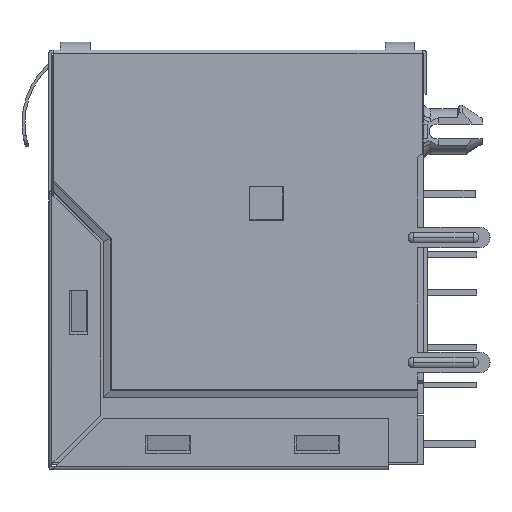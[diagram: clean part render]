
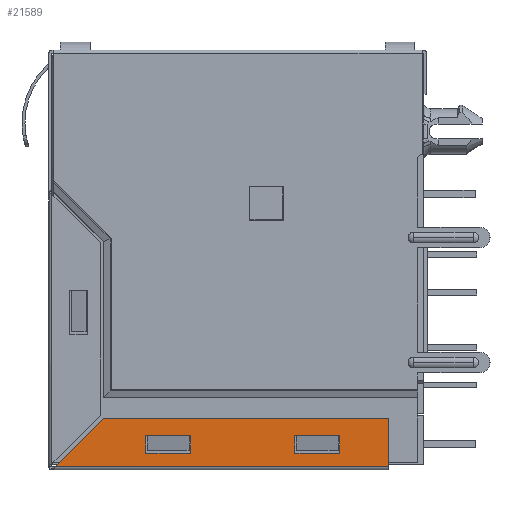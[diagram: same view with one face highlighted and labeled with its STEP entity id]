
A CAD part, left-side view. The second image highlights one B-rep face of the part: STEP entity #21589.
In plain terms, the highlighted planar face has unit normal (-1, 0, 0).
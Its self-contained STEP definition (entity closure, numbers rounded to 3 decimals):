
#802 = FACE_BOUND ( 'NONE', #19686, .T. ) ;
#1521 = VERTEX_POINT ( 'NONE', #7287 ) ;
#1597 = CARTESIAN_POINT ( 'NONE',  ( -31.88, 3.165, -25.58 ) ) ;
#2437 = ORIENTED_EDGE ( 'NONE', *, *, #51071, .T. ) ;
#3403 = CARTESIAN_POINT ( 'NONE',  ( -31.88, -6.835, -25.58 ) ) ;
#3561 = CARTESIAN_POINT ( 'NONE',  ( -31.88, -10.135, -27.67 ) ) ;
#5840 = CARTESIAN_POINT ( 'NONE',  ( -31.88, -10.135, -24.43 ) ) ;
#6438 = B_SPLINE_CURVE_WITH_KNOTS ( 'NONE', 1,
 ( #54370, #48683 ),
 .UNSPECIFIED., .F., .F.,
 ( 2, 2 ),
 ( 0., 1. ),
 .UNSPECIFIED. ) ;
#7287 = CARTESIAN_POINT ( 'NONE',  ( -31.88, -6.835, -26.78 ) ) ;
#7447 = B_SPLINE_CURVE_WITH_KNOTS ( 'NONE', 1,
 ( #21721, #28729 ),
 .UNSPECIFIED., .F., .F.,
 ( 2, 2 ),
 ( 0., 1. ),
 .UNSPECIFIED. ) ;
#9103 = CARTESIAN_POINT ( 'NONE',  ( -31.88, -6.835, -26.78 ) ) ;
#10113 = ORIENTED_EDGE ( 'NONE', *, *, #70867, .T. ) ;
#10382 = VERTEX_POINT ( 'NONE', #18526 ) ;
#10757 = VERTEX_POINT ( 'NONE', #53356 ) ;
#12150 = EDGE_LOOP ( 'NONE', ( #12982, #2437, #44208, #40241 ) ) ;
#12982 = ORIENTED_EDGE ( 'NONE', *, *, #63457, .T. ) ;
#13313 = CARTESIAN_POINT ( 'NONE',  ( -31.88, 6.165, -25.58 ) ) ;
#13814 = VERTEX_POINT ( 'NONE', #75172 ) ;
#15710 = CARTESIAN_POINT ( 'NONE',  ( -31.88, 9.005, -24.43 ) ) ;
#16967 = B_SPLINE_CURVE_WITH_KNOTS ( 'NONE', 1,
 ( #24337, #18397 ),
 .UNSPECIFIED., .F., .F.,
 ( 2, 2 ),
 ( 0., 1. ),
 .UNSPECIFIED. ) ;
#18397 = CARTESIAN_POINT ( 'NONE',  ( -31.88, -3.835, -26.78 ) ) ;
#18526 = CARTESIAN_POINT ( 'NONE',  ( -31.88, 12.245, -27.67 ) ) ;
#19686 = EDGE_LOOP ( 'NONE', ( #55014, #79416, #56093, #74237 ) ) ;
#20128 = CARTESIAN_POINT ( 'NONE',  ( -31.88, 6.165, -25.58 ) ) ;
#20222 = DIRECTION ( 'NONE',  ( -1., 0., 0. ) ) ;
#21165 = VERTEX_POINT ( 'NONE', #30728 ) ;
#21589 = ADVANCED_FACE ( 'NONE', ( #76416, #802, #34754 ), #44592, .T. ) ;
#21721 = CARTESIAN_POINT ( 'NONE',  ( -31.88, -3.835, -26.78 ) ) ;
#24337 = CARTESIAN_POINT ( 'NONE',  ( -31.88, -6.835, -26.78 ) ) ;
#25726 = VERTEX_POINT ( 'NONE', #26271 ) ;
#25918 = ORIENTED_EDGE ( 'NONE', *, *, #73327, .T. ) ;
#26271 = CARTESIAN_POINT ( 'NONE',  ( -31.88, -3.835, -26.78 ) ) ;
#28687 = EDGE_CURVE ( 'NONE', #77531, #10382, #40807, .T. ) ;
#28729 = CARTESIAN_POINT ( 'NONE',  ( -31.88, -3.835, -25.58 ) ) ;
#29521 = EDGE_LOOP ( 'NONE', ( #41422, #25918, #47184, #10113 ) ) ;
#30728 = CARTESIAN_POINT ( 'NONE',  ( -31.88, 6.165, -26.78 ) ) ;
#31362 = EDGE_CURVE ( 'NONE', #13814, #39121, #62130, .T. ) ;
#31887 = DIRECTION ( 'NONE',  ( 0., -1., 0. ) ) ;
#32704 = CARTESIAN_POINT ( 'NONE',  ( -31.88, 3.165, -26.78 ) ) ;
#33274 = CARTESIAN_POINT ( 'NONE',  ( -31.88, 3.165, -26.78 ) ) ;
#34106 = VERTEX_POINT ( 'NONE', #33274 ) ;
#34754 = FACE_BOUND ( 'NONE', #12150, .T. ) ;
#35662 = B_SPLINE_CURVE_WITH_KNOTS ( 'NONE', 1,
 ( #20128, #45288 ),
 .UNSPECIFIED., .F., .F.,
 ( 2, 2 ),
 ( 0., 1. ),
 .UNSPECIFIED. ) ;
#35679 = EDGE_CURVE ( 'NONE', #1521, #25726, #16967, .T. ) ;
#38654 = CARTESIAN_POINT ( 'NONE',  ( -31.88, 12.693, -27.79 ) ) ;
#39121 = VERTEX_POINT ( 'NONE', #46855 ) ;
#39978 = CARTESIAN_POINT ( 'NONE',  ( -31.88, -6.835, -25.58 ) ) ;
#40241 = ORIENTED_EDGE ( 'NONE', *, *, #46269, .T. ) ;
#40807 = B_SPLINE_CURVE_WITH_KNOTS ( 'NONE', 1,
 ( #76894, #77433 ),
 .UNSPECIFIED., .F., .F.,
 ( 2, 2 ),
 ( 0., 1. ),
 .UNSPECIFIED. ) ;
#41422 = ORIENTED_EDGE ( 'NONE', *, *, #68637, .F. ) ;
#41543 = B_SPLINE_CURVE_WITH_KNOTS ( 'NONE', 1,
 ( #5840, #79529 ),
 .UNSPECIFIED., .F., .F.,
 ( 2, 2 ),
 ( 0., 1. ),
 .UNSPECIFIED. ) ;
#42087 = B_SPLINE_CURVE_WITH_KNOTS ( 'NONE', 1,
 ( #68908, #44261 ),
 .UNSPECIFIED., .F., .F.,
 ( 2, 2 ),
 ( 0., 1. ),
 .UNSPECIFIED. ) ;
#43467 = B_SPLINE_CURVE_WITH_KNOTS ( 'NONE', 1,
 ( #49896, #68070 ),
 .UNSPECIFIED., .F., .F.,
 ( 2, 2 ),
 ( 0., 1. ),
 .UNSPECIFIED. ) ;
#44208 = ORIENTED_EDGE ( 'NONE', *, *, #78224, .T. ) ;
#44261 = CARTESIAN_POINT ( 'NONE',  ( -31.88, -10.135, -27.67 ) ) ;
#44592 = PLANE ( 'NONE',  #50009 ) ;
#45288 = CARTESIAN_POINT ( 'NONE',  ( -31.88, 3.165, -25.58 ) ) ;
#46269 = EDGE_CURVE ( 'NONE', #74099, #62589, #35662, .T. ) ;
#46855 = CARTESIAN_POINT ( 'NONE',  ( -31.88, -6.835, -25.58 ) ) ;
#46963 = CARTESIAN_POINT ( 'NONE',  ( -31.88, -3.835, -25.58 ) ) ;
#47184 = ORIENTED_EDGE ( 'NONE', *, *, #28687, .T. ) ;
#48239 = B_SPLINE_CURVE_WITH_KNOTS ( 'NONE', 1,
 ( #32704, #75795 ),
 .UNSPECIFIED., .F., .F.,
 ( 2, 2 ),
 ( 0., 1. ),
 .UNSPECIFIED. ) ;
#48683 = CARTESIAN_POINT ( 'NONE',  ( -31.88, 3.165, -26.78 ) ) ;
#49896 = CARTESIAN_POINT ( 'NONE',  ( -31.88, 6.165, -26.78 ) ) ;
#50009 = AXIS2_PLACEMENT_3D ( 'NONE', #38654, #20222, #31887 ) ;
#51071 = EDGE_CURVE ( 'NONE', #34106, #21165, #48239, .T. ) ;
#52400 = VECTOR ( 'NONE', #52593, 1000. ) ;
#52593 = DIRECTION ( 'NONE',  ( 0., -1., 0. ) ) ;
#53356 = CARTESIAN_POINT ( 'NONE',  ( -31.88, -10.135, -24.43 ) ) ;
#54370 = CARTESIAN_POINT ( 'NONE',  ( -31.88, 3.165, -25.58 ) ) ;
#55014 = ORIENTED_EDGE ( 'NONE', *, *, #77989, .T. ) ;
#56093 = ORIENTED_EDGE ( 'NONE', *, *, #61721, .T. ) ;
#56392 = LINE ( 'NONE', #60980, #52400 ) ;
#60980 = CARTESIAN_POINT ( 'NONE',  ( -31.88, 1.055, -27.67 ) ) ;
#61721 = EDGE_CURVE ( 'NONE', #25726, #13814, #7447, .T. ) ;
#62130 = B_SPLINE_CURVE_WITH_KNOTS ( 'NONE', 1,
 ( #46963, #3403 ),
 .UNSPECIFIED., .F., .F.,
 ( 2, 2 ),
 ( 0., 1. ),
 .UNSPECIFIED. ) ;
#62589 = VERTEX_POINT ( 'NONE', #1597 ) ;
#62663 = VERTEX_POINT ( 'NONE', #3561 ) ;
#63457 = EDGE_CURVE ( 'NONE', #62589, #34106, #6438, .T. ) ;
#63818 = B_SPLINE_CURVE_WITH_KNOTS ( 'NONE', 1,
 ( #39978, #9103 ),
 .UNSPECIFIED., .F., .F.,
 ( 2, 2 ),
 ( 0., 1. ),
 .UNSPECIFIED. ) ;
#68070 = CARTESIAN_POINT ( 'NONE',  ( -31.88, 6.165, -25.58 ) ) ;
#68637 = EDGE_CURVE ( 'NONE', #10757, #62663, #42087, .T. ) ;
#68908 = CARTESIAN_POINT ( 'NONE',  ( -31.88, -10.135, -24.43 ) ) ;
#70867 = EDGE_CURVE ( 'NONE', #10382, #62663, #56392, .T. ) ;
#73327 = EDGE_CURVE ( 'NONE', #10757, #77531, #41543, .T. ) ;
#74099 = VERTEX_POINT ( 'NONE', #13313 ) ;
#74237 = ORIENTED_EDGE ( 'NONE', *, *, #31362, .T. ) ;
#75172 = CARTESIAN_POINT ( 'NONE',  ( -31.88, -3.835, -25.58 ) ) ;
#75795 = CARTESIAN_POINT ( 'NONE',  ( -31.88, 6.165, -26.78 ) ) ;
#76416 = FACE_OUTER_BOUND ( 'NONE', #29521, .T. ) ;
#76894 = CARTESIAN_POINT ( 'NONE',  ( -31.88, 9.005, -24.43 ) ) ;
#77433 = CARTESIAN_POINT ( 'NONE',  ( -31.88, 12.245, -27.67 ) ) ;
#77531 = VERTEX_POINT ( 'NONE', #15710 ) ;
#77989 = EDGE_CURVE ( 'NONE', #39121, #1521, #63818, .T. ) ;
#78224 = EDGE_CURVE ( 'NONE', #21165, #74099, #43467, .T. ) ;
#79416 = ORIENTED_EDGE ( 'NONE', *, *, #35679, .T. ) ;
#79529 = CARTESIAN_POINT ( 'NONE',  ( -31.88, 9.005, -24.43 ) ) ;
